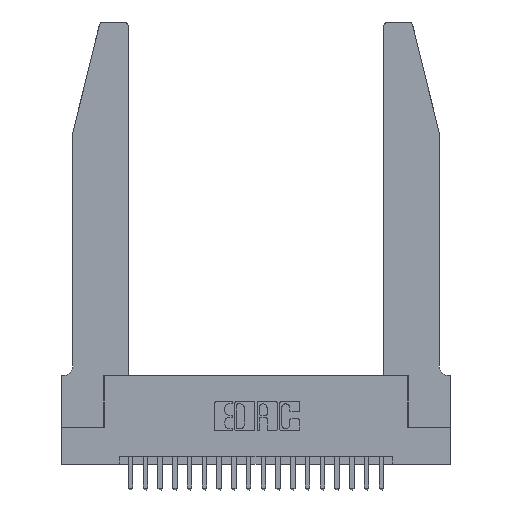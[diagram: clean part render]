
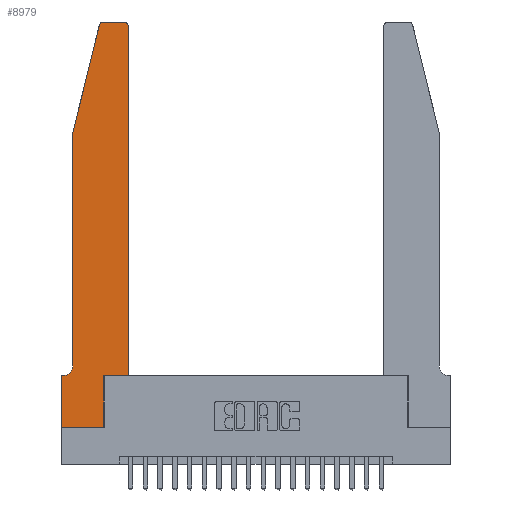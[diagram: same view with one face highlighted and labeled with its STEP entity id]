
A CAD part, top view. The second image highlights one B-rep face of the part: STEP entity #8979.
In plain terms, the highlighted planar face has unit normal (0, 0, 1).
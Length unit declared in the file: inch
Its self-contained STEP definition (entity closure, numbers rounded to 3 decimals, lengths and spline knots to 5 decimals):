
#26 = DIRECTION ( 'NONE',  ( 0., 1., 0. ) ) ;
#412 = CARTESIAN_POINT ( 'NONE',  ( 0., 0., 0.37 ) ) ;
#673 = VERTEX_POINT ( 'NONE', #13271 ) ;
#952 = VERTEX_POINT ( 'NONE', #2526 ) ;
#1252 = VERTEX_POINT ( 'NONE', #19228 ) ;
#1269 = DIRECTION ( 'NONE',  ( 1., 0., 0. ) ) ;
#1495 = LINE ( 'NONE', #16216, #14742 ) ;
#1614 = EDGE_CURVE ( 'NONE', #20080, #673, #18469, .T. ) ;
#1793 = DIRECTION ( 'NONE',  ( 1., 0., 0. ) ) ;
#1978 = CIRCLE ( 'NONE', #4656, 0.07 ) ;
#2039 = CARTESIAN_POINT ( 'NONE',  ( 0.0755, 2., 0.37 ) ) ;
#2448 = EDGE_LOOP ( 'NONE', ( #5254, #14191, #14646, #22239, #15397, #12843, #13829, #17799, #8967, #8146, #18998, #11198 ) ) ;
#2484 = VERTEX_POINT ( 'NONE', #10376 ) ;
#2509 = EDGE_CURVE ( 'NONE', #15705, #8856, #6966, .T. ) ;
#2526 = CARTESIAN_POINT ( 'NONE',  ( 0.0755, 2., 0.37 ) ) ;
#3319 = DIRECTION ( 'NONE',  ( 0., 1., 0. ) ) ;
#3449 = VECTOR ( 'NONE', #10425, 39.37008 ) ;
#3644 = DIRECTION ( 'NONE',  ( 1., 0., 0. ) ) ;
#3916 = AXIS2_PLACEMENT_3D ( 'NONE', #21170, #12121, #1793 ) ;
#4170 = VERTEX_POINT ( 'NONE', #6451 ) ;
#4431 = VECTOR ( 'NONE', #12353, 39.37008 ) ;
#4656 = AXIS2_PLACEMENT_3D ( 'NONE', #9714, #21605, #11436 ) ;
#5254 = ORIENTED_EDGE ( 'NONE', *, *, #10868, .T. ) ;
#5316 = CARTESIAN_POINT ( 'NONE',  ( 0.4505, 0.35, 0.37 ) ) ;
#5319 = EDGE_CURVE ( 'NONE', #18496, #14933, #14373, .T. ) ;
#5737 = EDGE_CURVE ( 'NONE', #4170, #1252, #1978, .T. ) ;
#6148 = CARTESIAN_POINT ( 'NONE',  ( 0.4205, 2.72, 0.37 ) ) ;
#6451 = CARTESIAN_POINT ( 'NONE',  ( 0.0755, 0.42, 0.37 ) ) ;
#6535 = VECTOR ( 'NONE', #3644, 39.37008 ) ;
#6645 = VECTOR ( 'NONE', #13705, 39.37008 ) ;
#6778 = CARTESIAN_POINT ( 'NONE',  ( 0.2605, 2.75, 0.37 ) ) ;
#6966 = LINE ( 'NONE', #5316, #15047 ) ;
#7322 = EDGE_CURVE ( 'NONE', #14242, #15705, #15664, .T. ) ;
#7334 = DIRECTION ( 'NONE',  ( -0.239, -0.971, 0. ) ) ;
#7876 = DIRECTION ( 'NONE',  ( 1., 0., 0. ) ) ;
#8146 = ORIENTED_EDGE ( 'NONE', *, *, #7322, .T. ) ;
#8483 = CARTESIAN_POINT ( 'NONE',  ( 0., 0.35, 0.37 ) ) ;
#8551 = CARTESIAN_POINT ( 'NONE',  ( 0.2865, 0.35, 0.37 ) ) ;
#8856 = VERTEX_POINT ( 'NONE', #16516 ) ;
#8967 = ORIENTED_EDGE ( 'NONE', *, *, #14228, .T. ) ;
#8979 = ADVANCED_FACE ( 'NONE', ( #20348 ), #20407, .T. ) ;
#9651 = EDGE_CURVE ( 'NONE', #16621, #20080, #12600, .T. ) ;
#9714 = CARTESIAN_POINT ( 'NONE',  ( 0.0055, 0.42, 0.37 ) ) ;
#9984 = EDGE_CURVE ( 'NONE', #1252, #16621, #1495, .T. ) ;
#10064 = CIRCLE ( 'NONE', #16807, 0.03 ) ;
#10376 = CARTESIAN_POINT ( 'NONE',  ( 0.4205, 2.75, 0.37 ) ) ;
#10425 = DIRECTION ( 'NONE',  ( 0., -1., 0. ) ) ;
#10752 = CARTESIAN_POINT ( 'NONE',  ( 0.0755, 2., 0.37 ) ) ;
#10868 = EDGE_CURVE ( 'NONE', #2484, #18496, #20781, .T. ) ;
#11198 = ORIENTED_EDGE ( 'NONE', *, *, #11896, .T. ) ;
#11436 = DIRECTION ( 'NONE',  ( -1., 0., 0. ) ) ;
#11896 = EDGE_CURVE ( 'NONE', #8856, #2484, #10064, .T. ) ;
#11906 = DIRECTION ( 'NONE',  ( 1., 0., 0. ) ) ;
#12121 = DIRECTION ( 'NONE',  ( 0., 0., 1. ) ) ;
#12214 = CARTESIAN_POINT ( 'NONE',  ( 0.4505, 0.35, 0.37 ) ) ;
#12353 = DIRECTION ( 'NONE',  ( 0., -1., 0. ) ) ;
#12502 = EDGE_CURVE ( 'NONE', #952, #4170, #13561, .T. ) ;
#12600 = LINE ( 'NONE', #21028, #3449 ) ;
#12843 = ORIENTED_EDGE ( 'NONE', *, *, #9984, .T. ) ;
#13271 = CARTESIAN_POINT ( 'NONE',  ( 0.2865, 0., 0.37 ) ) ;
#13305 = CARTESIAN_POINT ( 'NONE',  ( 0., 0., 0.37 ) ) ;
#13561 = LINE ( 'NONE', #2039, #4431 ) ;
#13632 = CARTESIAN_POINT ( 'NONE',  ( 0.284, 2.75, 0.37 ) ) ;
#13651 = CARTESIAN_POINT ( 'NONE',  ( 0.2865, 0.35, 0.37 ) ) ;
#13700 = CARTESIAN_POINT ( 'NONE',  ( 0.25487, 2.72718, 0.37 ) ) ;
#13705 = DIRECTION ( 'NONE',  ( -1., 0., 0. ) ) ;
#13829 = ORIENTED_EDGE ( 'NONE', *, *, #9651, .T. ) ;
#14010 = VECTOR ( 'NONE', #1269, 39.37008 ) ;
#14191 = ORIENTED_EDGE ( 'NONE', *, *, #5319, .T. ) ;
#14228 = EDGE_CURVE ( 'NONE', #673, #14242, #19344, .T. ) ;
#14242 = VERTEX_POINT ( 'NONE', #8551 ) ;
#14373 = CIRCLE ( 'NONE', #3916, 0.03 ) ;
#14646 = ORIENTED_EDGE ( 'NONE', *, *, #17476, .T. ) ;
#14742 = VECTOR ( 'NONE', #16149, 39.37008 ) ;
#14933 = VERTEX_POINT ( 'NONE', #13700 ) ;
#15047 = VECTOR ( 'NONE', #26, 39.37008 ) ;
#15397 = ORIENTED_EDGE ( 'NONE', *, *, #5737, .T. ) ;
#15640 = AXIS2_PLACEMENT_3D ( 'NONE', #8483, #22049, #11906 ) ;
#15664 = LINE ( 'NONE', #12214, #6535 ) ;
#15705 = VERTEX_POINT ( 'NONE', #16192 ) ;
#15945 = VECTOR ( 'NONE', #3319, 39.37008 ) ;
#16149 = DIRECTION ( 'NONE',  ( -1., 0., 0. ) ) ;
#16192 = CARTESIAN_POINT ( 'NONE',  ( 0.4505, 0.35, 0.37 ) ) ;
#16216 = CARTESIAN_POINT ( 'NONE',  ( 0.0755, 0.35, 0.37 ) ) ;
#16516 = CARTESIAN_POINT ( 'NONE',  ( 0.4505, 2.72, 0.37 ) ) ;
#16621 = VERTEX_POINT ( 'NONE', #21792 ) ;
#16636 = LINE ( 'NONE', #10752, #20056 ) ;
#16807 = AXIS2_PLACEMENT_3D ( 'NONE', #6148, #18064, #7876 ) ;
#17476 = EDGE_CURVE ( 'NONE', #14933, #952, #16636, .T. ) ;
#17799 = ORIENTED_EDGE ( 'NONE', *, *, #1614, .T. ) ;
#18064 = DIRECTION ( 'NONE',  ( 0., 0., 1. ) ) ;
#18469 = LINE ( 'NONE', #13305, #14010 ) ;
#18496 = VERTEX_POINT ( 'NONE', #13632 ) ;
#18998 = ORIENTED_EDGE ( 'NONE', *, *, #2509, .T. ) ;
#19228 = CARTESIAN_POINT ( 'NONE',  ( 0.0055, 0.35, 0.37 ) ) ;
#19344 = LINE ( 'NONE', #13651, #15945 ) ;
#20056 = VECTOR ( 'NONE', #7334, 39.37008 ) ;
#20080 = VERTEX_POINT ( 'NONE', #412 ) ;
#20348 = FACE_OUTER_BOUND ( 'NONE', #2448, .T. ) ;
#20407 = PLANE ( 'NONE',  #15640 ) ;
#20781 = LINE ( 'NONE', #6778, #6645 ) ;
#21028 = CARTESIAN_POINT ( 'NONE',  ( 0., 0., 0.37 ) ) ;
#21170 = CARTESIAN_POINT ( 'NONE',  ( 0.284, 2.72, 0.37 ) ) ;
#21605 = DIRECTION ( 'NONE',  ( 0., 0., -1. ) ) ;
#21792 = CARTESIAN_POINT ( 'NONE',  ( 0., 0.35, 0.37 ) ) ;
#22049 = DIRECTION ( 'NONE',  ( 0., 0., 1. ) ) ;
#22239 = ORIENTED_EDGE ( 'NONE', *, *, #12502, .T. ) ;
